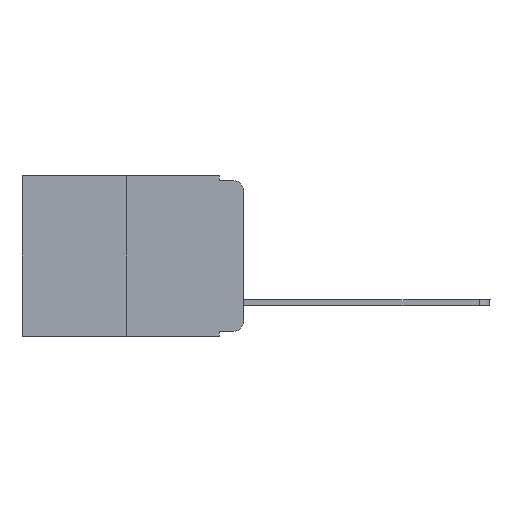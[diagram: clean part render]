
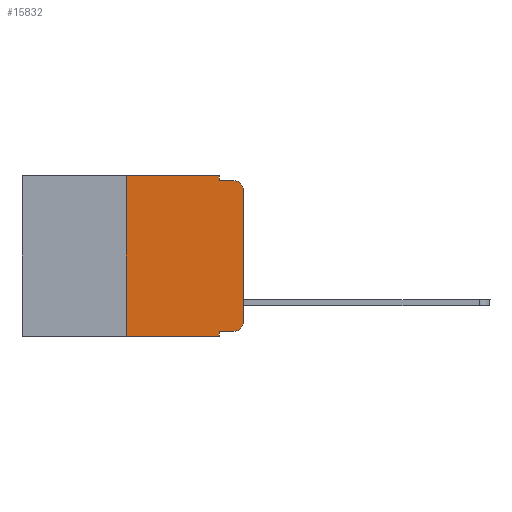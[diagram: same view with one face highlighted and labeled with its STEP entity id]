
A CAD part, left-side view. The second image highlights one B-rep face of the part: STEP entity #15832.
In plain terms, the highlighted planar face has unit normal (-1, 0, 0).
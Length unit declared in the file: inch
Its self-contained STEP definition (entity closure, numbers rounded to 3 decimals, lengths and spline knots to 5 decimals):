
#419 = DIRECTION ( 'NONE',  ( 0., 0., -1. ) ) ;
#553 = CARTESIAN_POINT ( 'NONE',  ( 0., 0.051, -0.343 ) ) ;
#961 = EDGE_CURVE ( 'NONE', #4497, #6391, #11105, .T. ) ;
#1082 = LINE ( 'NONE', #14401, #8028 ) ;
#1162 = LINE ( 'NONE', #9642, #7453 ) ;
#1319 = DIRECTION ( 'NONE',  ( 0., 0., -1. ) ) ;
#1484 = FACE_OUTER_BOUND ( 'NONE', #7497, .T. ) ;
#1517 = CARTESIAN_POINT ( 'NONE',  ( 0., 0.473, -0.343 ) ) ;
#1548 = CARTESIAN_POINT ( 'NONE',  ( 0., 0., 0. ) ) ;
#1593 = CARTESIAN_POINT ( 'NONE',  ( 0., 0.02, -0.333 ) ) ;
#1638 = VERTEX_POINT ( 'NONE', #12522 ) ;
#1839 = EDGE_CURVE ( 'NONE', #15274, #6391, #9456, .T. ) ;
#2347 = CARTESIAN_POINT ( 'NONE',  ( 0., 0.051, -0.01 ) ) ;
#2434 = CARTESIAN_POINT ( 'NONE',  ( 0., 0.25, -0.343 ) ) ;
#2713 = ORIENTED_EDGE ( 'NONE', *, *, #1839, .F. ) ;
#2911 = CARTESIAN_POINT ( 'NONE',  ( 0., 0.02, -0.313 ) ) ;
#3092 = CARTESIAN_POINT ( 'NONE',  ( 0., 0.051, -0.01 ) ) ;
#3123 = CIRCLE ( 'NONE', #5182, 0.02 ) ;
#3173 = LINE ( 'NONE', #3092, #13025 ) ;
#3301 = VERTEX_POINT ( 'NONE', #9788 ) ;
#3624 = ORIENTED_EDGE ( 'NONE', *, *, #5231, .F. ) ;
#3899 = CARTESIAN_POINT ( 'NONE',  ( 0., 0.02, -0.03 ) ) ;
#4062 = DIRECTION ( 'NONE',  ( 0., 0., -1. ) ) ;
#4094 = AXIS2_PLACEMENT_3D ( 'NONE', #9876, #12454, #1319 ) ;
#4497 = VERTEX_POINT ( 'NONE', #2434 ) ;
#4644 = EDGE_CURVE ( 'NONE', #9562, #12323, #3123, .T. ) ;
#5182 = AXIS2_PLACEMENT_3D ( 'NONE', #2911, #11401, #419 ) ;
#5231 = EDGE_CURVE ( 'NONE', #3301, #10376, #1162, .T. ) ;
#5316 = VECTOR ( 'NONE', #12569, 39.37008 ) ;
#5592 = ORIENTED_EDGE ( 'NONE', *, *, #4644, .T. ) ;
#5668 = EDGE_CURVE ( 'NONE', #15274, #9562, #7005, .T. ) ;
#5877 = CARTESIAN_POINT ( 'NONE',  ( 0., 0.051, -0.333 ) ) ;
#6153 = LINE ( 'NONE', #11026, #11416 ) ;
#6391 = VERTEX_POINT ( 'NONE', #553 ) ;
#7005 = LINE ( 'NONE', #5877, #13558 ) ;
#7290 = ORIENTED_EDGE ( 'NONE', *, *, #14204, .F. ) ;
#7422 = CARTESIAN_POINT ( 'NONE',  ( 0., 0.02, -0.01 ) ) ;
#7453 = VECTOR ( 'NONE', #9491, 39.37008 ) ;
#7497 = EDGE_LOOP ( 'NONE', ( #8411, #7615, #7290, #11381, #3624, #13690, #10891, #2713, #13574, #5592 ) ) ;
#7615 = ORIENTED_EDGE ( 'NONE', *, *, #7904, .T. ) ;
#7715 = PLANE ( 'NONE',  #4094 ) ;
#7904 = EDGE_CURVE ( 'NONE', #1638, #11263, #12372, .T. ) ;
#8028 = VECTOR ( 'NONE', #8283, 39.37008 ) ;
#8213 = EDGE_CURVE ( 'NONE', #10376, #10247, #1082, .T. ) ;
#8283 = DIRECTION ( 'NONE',  ( 0., 0., -1. ) ) ;
#8411 = ORIENTED_EDGE ( 'NONE', *, *, #14492, .T. ) ;
#8561 = DIRECTION ( 'NONE',  ( 0., 0., -1. ) ) ;
#8778 = AXIS2_PLACEMENT_3D ( 'NONE', #3899, #11171, #4062 ) ;
#9456 = LINE ( 'NONE', #15797, #11794 ) ;
#9491 = DIRECTION ( 'NONE',  ( 0., -1., 0. ) ) ;
#9562 = VERTEX_POINT ( 'NONE', #1593 ) ;
#9642 = CARTESIAN_POINT ( 'NONE',  ( 0., 0.473, 0. ) ) ;
#9788 = CARTESIAN_POINT ( 'NONE',  ( 0., 0.25, 0. ) ) ;
#9876 = CARTESIAN_POINT ( 'NONE',  ( 0., 0.473, 0. ) ) ;
#10247 = VERTEX_POINT ( 'NONE', #2347 ) ;
#10376 = VERTEX_POINT ( 'NONE', #15180 ) ;
#10765 = DIRECTION ( 'NONE',  ( 0., -1., 0. ) ) ;
#10891 = ORIENTED_EDGE ( 'NONE', *, *, #961, .T. ) ;
#11026 = CARTESIAN_POINT ( 'NONE',  ( 0., 0.25, 0. ) ) ;
#11105 = LINE ( 'NONE', #1517, #5316 ) ;
#11171 = DIRECTION ( 'NONE',  ( -1., 0., 0. ) ) ;
#11263 = VERTEX_POINT ( 'NONE', #7422 ) ;
#11381 = ORIENTED_EDGE ( 'NONE', *, *, #8213, .F. ) ;
#11401 = DIRECTION ( 'NONE',  ( -1., 0., 0. ) ) ;
#11416 = VECTOR ( 'NONE', #14976, 39.37008 ) ;
#11794 = VECTOR ( 'NONE', #8561, 39.37008 ) ;
#12323 = VERTEX_POINT ( 'NONE', #15771 ) ;
#12372 = CIRCLE ( 'NONE', #8778, 0.02 ) ;
#12431 = EDGE_CURVE ( 'NONE', #4497, #3301, #6153, .T. ) ;
#12454 = DIRECTION ( 'NONE',  ( 1., 0., 0. ) ) ;
#12522 = CARTESIAN_POINT ( 'NONE',  ( 0., 0., -0.03 ) ) ;
#12569 = DIRECTION ( 'NONE',  ( 0., -1., 0. ) ) ;
#12596 = DIRECTION ( 'NONE',  ( 0., 0., 1. ) ) ;
#12637 = DIRECTION ( 'NONE',  ( 0., -1., 0. ) ) ;
#13025 = VECTOR ( 'NONE', #12637, 39.37008 ) ;
#13034 = VECTOR ( 'NONE', #12596, 39.37008 ) ;
#13558 = VECTOR ( 'NONE', #10765, 39.37008 ) ;
#13574 = ORIENTED_EDGE ( 'NONE', *, *, #5668, .T. ) ;
#13690 = ORIENTED_EDGE ( 'NONE', *, *, #12431, .F. ) ;
#13718 = LINE ( 'NONE', #1548, #13034 ) ;
#14204 = EDGE_CURVE ( 'NONE', #10247, #11263, #3173, .T. ) ;
#14401 = CARTESIAN_POINT ( 'NONE',  ( 0., 0.051, 0. ) ) ;
#14492 = EDGE_CURVE ( 'NONE', #12323, #1638, #13718, .T. ) ;
#14665 = CARTESIAN_POINT ( 'NONE',  ( 0., 0.051, -0.333 ) ) ;
#14976 = DIRECTION ( 'NONE',  ( 0., 0., 1. ) ) ;
#15180 = CARTESIAN_POINT ( 'NONE',  ( 0., 0.051, 0. ) ) ;
#15274 = VERTEX_POINT ( 'NONE', #14665 ) ;
#15771 = CARTESIAN_POINT ( 'NONE',  ( 0., 0., -0.313 ) ) ;
#15797 = CARTESIAN_POINT ( 'NONE',  ( 0., 0.051, 0. ) ) ;
#15832 = ADVANCED_FACE ( 'NONE', ( #1484 ), #7715, .F. ) ;
